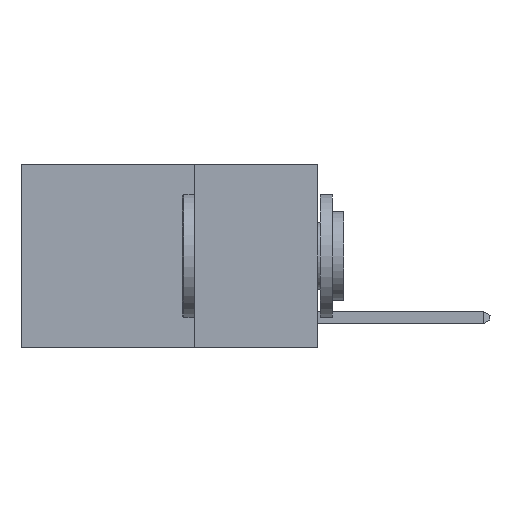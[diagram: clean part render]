
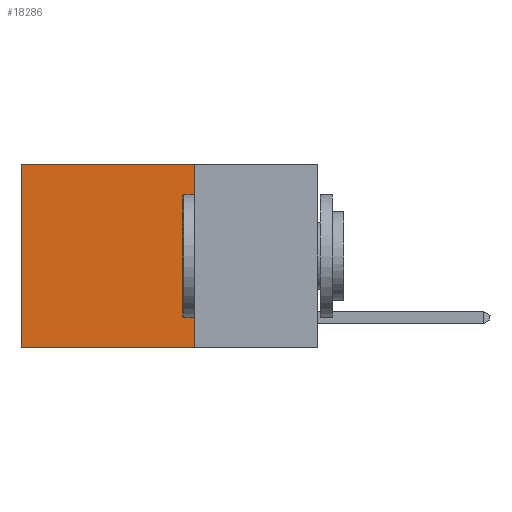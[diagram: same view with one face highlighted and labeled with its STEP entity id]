
A CAD part, left-side view. The second image highlights one B-rep face of the part: STEP entity #18286.
In plain terms, the highlighted planar face has unit normal (-1, 0, 0).
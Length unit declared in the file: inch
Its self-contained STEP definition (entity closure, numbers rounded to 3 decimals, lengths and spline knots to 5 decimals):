
#89 = LINE ( 'NONE', #8805, #16430 ) ;
#374 = ORIENTED_EDGE ( 'NONE', *, *, #18429, .F. ) ;
#381 = CARTESIAN_POINT ( 'NONE',  ( 0.2625, 0.25, -0.37 ) ) ;
#511 = EDGE_LOOP ( 'NONE', ( #11782, #14684, #374, #6451 ) ) ;
#532 = EDGE_CURVE ( 'NONE', #11966, #16837, #1075, .T. ) ;
#889 = AXIS2_PLACEMENT_3D ( 'NONE', #4558, #17186, #7778 ) ;
#1046 = LINE ( 'NONE', #8436, #17360 ) ;
#1075 = LINE ( 'NONE', #381, #16902 ) ;
#1824 = LINE ( 'NONE', #2862, #9772 ) ;
#2862 = CARTESIAN_POINT ( 'NONE',  ( 0.2625, 0.6, 0. ) ) ;
#4058 = DIRECTION ( 'NONE',  ( 0., 1., 0. ) ) ;
#4558 = CARTESIAN_POINT ( 'NONE',  ( 0.2625, 0.25, 0. ) ) ;
#5766 = CARTESIAN_POINT ( 'NONE',  ( 0.2625, 0.25, -0.37 ) ) ;
#6357 = EDGE_CURVE ( 'NONE', #19519, #8748, #89, .T. ) ;
#6451 = ORIENTED_EDGE ( 'NONE', *, *, #6357, .T. ) ;
#6534 = EDGE_CURVE ( 'NONE', #8748, #16837, #1824, .T. ) ;
#6919 = CARTESIAN_POINT ( 'NONE',  ( 0.2625, 0.6, -0.37 ) ) ;
#7778 = DIRECTION ( 'NONE',  ( 0., 0., -1. ) ) ;
#8277 = FACE_OUTER_BOUND ( 'NONE', #511, .T. ) ;
#8436 = CARTESIAN_POINT ( 'NONE',  ( 0.2625, 0.25, 0. ) ) ;
#8748 = VERTEX_POINT ( 'NONE', #10367 ) ;
#8805 = CARTESIAN_POINT ( 'NONE',  ( 0.2625, 0.25, 0. ) ) ;
#9202 = DIRECTION ( 'NONE',  ( 0., 0., -1. ) ) ;
#9772 = VECTOR ( 'NONE', #9202, 39.37008 ) ;
#10367 = CARTESIAN_POINT ( 'NONE',  ( 0.2625, 0.6, 0. ) ) ;
#11591 = DIRECTION ( 'NONE',  ( 0., 0., -1. ) ) ;
#11782 = ORIENTED_EDGE ( 'NONE', *, *, #6534, .T. ) ;
#11966 = VERTEX_POINT ( 'NONE', #5766 ) ;
#12999 = CARTESIAN_POINT ( 'NONE',  ( 0.2625, 0.25, 0. ) ) ;
#14026 = PLANE ( 'NONE',  #889 ) ;
#14684 = ORIENTED_EDGE ( 'NONE', *, *, #532, .F. ) ;
#16430 = VECTOR ( 'NONE', #4058, 39.37008 ) ;
#16837 = VERTEX_POINT ( 'NONE', #6919 ) ;
#16902 = VECTOR ( 'NONE', #17205, 39.37008 ) ;
#17186 = DIRECTION ( 'NONE',  ( 1., 0., 0. ) ) ;
#17205 = DIRECTION ( 'NONE',  ( 0., 1., 0. ) ) ;
#17360 = VECTOR ( 'NONE', #11591, 39.37008 ) ;
#18286 = ADVANCED_FACE ( 'NONE', ( #8277 ), #14026, .F. ) ;
#18429 = EDGE_CURVE ( 'NONE', #19519, #11966, #1046, .T. ) ;
#19519 = VERTEX_POINT ( 'NONE', #12999 ) ;
